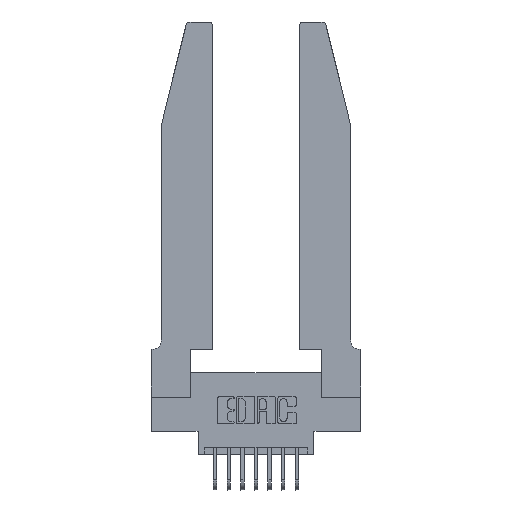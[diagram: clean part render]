
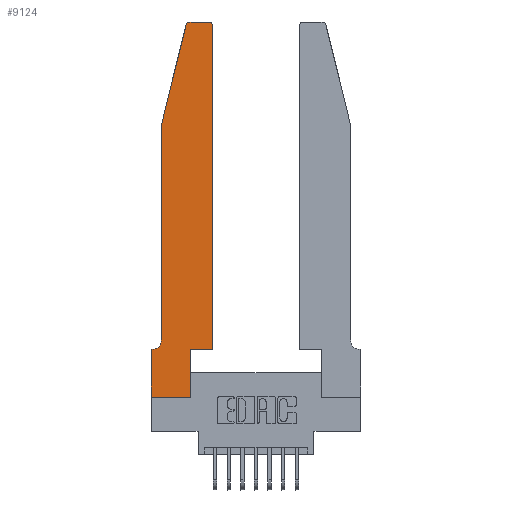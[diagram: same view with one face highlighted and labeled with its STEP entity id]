
A CAD part, top view. The second image highlights one B-rep face of the part: STEP entity #9124.
In plain terms, the highlighted planar face has unit normal (0, 0, 1).
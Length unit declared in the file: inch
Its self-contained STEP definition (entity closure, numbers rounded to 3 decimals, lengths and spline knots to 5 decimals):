
#321 = CARTESIAN_POINT ( 'NONE',  ( 0.0755, 2., 0.37 ) ) ;
#532 = DIRECTION ( 'NONE',  ( -0.239, -0.971, 0. ) ) ;
#691 = DIRECTION ( 'NONE',  ( 1., 0., 0. ) ) ;
#739 = FACE_OUTER_BOUND ( 'NONE', #866, .T. ) ;
#762 = ORIENTED_EDGE ( 'NONE', *, *, #8287, .T. ) ;
#866 = EDGE_LOOP ( 'NONE', ( #4754, #2908, #10912, #8141, #12727, #3979, #762, #2151, #1690, #1824, #6957, #2528 ) ) ;
#906 = EDGE_CURVE ( 'NONE', #6568, #2454, #1935, .T. ) ;
#1065 = AXIS2_PLACEMENT_3D ( 'NONE', #1657, #1554, #691 ) ;
#1554 = DIRECTION ( 'NONE',  ( 0., 0., 1. ) ) ;
#1657 = CARTESIAN_POINT ( 'NONE',  ( 0.284, 2.72, 0.37 ) ) ;
#1690 = ORIENTED_EDGE ( 'NONE', *, *, #4839, .T. ) ;
#1824 = ORIENTED_EDGE ( 'NONE', *, *, #3518, .T. ) ;
#1935 = LINE ( 'NONE', #15630, #15192 ) ;
#2151 = ORIENTED_EDGE ( 'NONE', *, *, #6370, .T. ) ;
#2232 = DIRECTION ( 'NONE',  ( 0., 0., -1. ) ) ;
#2344 = DIRECTION ( 'NONE',  ( 1., 0., 0. ) ) ;
#2454 = VERTEX_POINT ( 'NONE', #4902 ) ;
#2528 = ORIENTED_EDGE ( 'NONE', *, *, #13928, .T. ) ;
#2529 = EDGE_CURVE ( 'NONE', #5064, #13050, #14979, .T. ) ;
#2542 = AXIS2_PLACEMENT_3D ( 'NONE', #3660, #16476, #8797 ) ;
#2670 = LINE ( 'NONE', #3162, #9095 ) ;
#2908 = ORIENTED_EDGE ( 'NONE', *, *, #2529, .T. ) ;
#2967 = DIRECTION ( 'NONE',  ( 0., 0., 1. ) ) ;
#3162 = CARTESIAN_POINT ( 'NONE',  ( 0.0755, 2., 0.37 ) ) ;
#3518 = EDGE_CURVE ( 'NONE', #9784, #12158, #11514, .T. ) ;
#3660 = CARTESIAN_POINT ( 'NONE',  ( 0., 0.35, 0.37 ) ) ;
#3701 = LINE ( 'NONE', #15547, #13466 ) ;
#3979 = ORIENTED_EDGE ( 'NONE', *, *, #906, .T. ) ;
#3990 = DIRECTION ( 'NONE',  ( 1., 0., 0. ) ) ;
#4153 = LINE ( 'NONE', #8307, #13906 ) ;
#4227 = DIRECTION ( 'NONE',  ( 0., 1., 0. ) ) ;
#4754 = ORIENTED_EDGE ( 'NONE', *, *, #16108, .T. ) ;
#4839 = EDGE_CURVE ( 'NONE', #8522, #9784, #3701, .T. ) ;
#4902 = CARTESIAN_POINT ( 'NONE',  ( 0., 0.35, 0.37 ) ) ;
#5064 = VERTEX_POINT ( 'NONE', #5830 ) ;
#5167 = VECTOR ( 'NONE', #2344, 39.37008 ) ;
#5707 = VECTOR ( 'NONE', #6955, 39.37008 ) ;
#5830 = CARTESIAN_POINT ( 'NONE',  ( 0.284, 2.75, 0.37 ) ) ;
#5882 = LINE ( 'NONE', #12896, #12227 ) ;
#6125 = AXIS2_PLACEMENT_3D ( 'NONE', #9896, #2232, #11203 ) ;
#6370 = EDGE_CURVE ( 'NONE', #12316, #8522, #5882, .T. ) ;
#6496 = VERTEX_POINT ( 'NONE', #8105 ) ;
#6568 = VERTEX_POINT ( 'NONE', #15944 ) ;
#6630 = DIRECTION ( 'NONE',  ( 0., 1., 0. ) ) ;
#6821 = CARTESIAN_POINT ( 'NONE',  ( 0.4505, 0.35, 0.37 ) ) ;
#6955 = DIRECTION ( 'NONE',  ( 0., -1., 0. ) ) ;
#6957 = ORIENTED_EDGE ( 'NONE', *, *, #11340, .T. ) ;
#7007 = LINE ( 'NONE', #6821, #12957 ) ;
#7086 = CARTESIAN_POINT ( 'NONE',  ( 0.25487, 2.72718, 0.37 ) ) ;
#7095 = EDGE_CURVE ( 'NONE', #13050, #7576, #2670, .T. ) ;
#7122 = CARTESIAN_POINT ( 'NONE',  ( 0.0755, 0.42, 0.37 ) ) ;
#7249 = AXIS2_PLACEMENT_3D ( 'NONE', #10598, #2967, #11891 ) ;
#7576 = VERTEX_POINT ( 'NONE', #321 ) ;
#8105 = CARTESIAN_POINT ( 'NONE',  ( 0.4505, 2.72, 0.37 ) ) ;
#8141 = ORIENTED_EDGE ( 'NONE', *, *, #12514, .T. ) ;
#8287 = EDGE_CURVE ( 'NONE', #2454, #12316, #9082, .T. ) ;
#8307 = CARTESIAN_POINT ( 'NONE',  ( 0.0755, 2., 0.37 ) ) ;
#8459 = EDGE_CURVE ( 'NONE', #12044, #6568, #16489, .T. ) ;
#8522 = VERTEX_POINT ( 'NONE', #15077 ) ;
#8783 = DIRECTION ( 'NONE',  ( -1., 0., 0. ) ) ;
#8797 = DIRECTION ( 'NONE',  ( 1., 0., 0. ) ) ;
#8838 = DIRECTION ( 'NONE',  ( -1., 0., 0. ) ) ;
#9082 = LINE ( 'NONE', #15887, #5707 ) ;
#9095 = VECTOR ( 'NONE', #532, 39.37008 ) ;
#9124 = ADVANCED_FACE ( 'NONE', ( #739 ), #16419, .T. ) ;
#9158 = VECTOR ( 'NONE', #8783, 39.37008 ) ;
#9535 = VERTEX_POINT ( 'NONE', #13343 ) ;
#9577 = DIRECTION ( 'NONE',  ( 0., -1., 0. ) ) ;
#9784 = VERTEX_POINT ( 'NONE', #13885 ) ;
#9896 = CARTESIAN_POINT ( 'NONE',  ( 0.0055, 0.42, 0.37 ) ) ;
#10004 = CARTESIAN_POINT ( 'NONE',  ( 0.4505, 0.35, 0.37 ) ) ;
#10598 = CARTESIAN_POINT ( 'NONE',  ( 0.4205, 2.72, 0.37 ) ) ;
#10912 = ORIENTED_EDGE ( 'NONE', *, *, #7095, .T. ) ;
#11203 = DIRECTION ( 'NONE',  ( -1., 0., 0. ) ) ;
#11340 = EDGE_CURVE ( 'NONE', #12158, #6496, #7007, .T. ) ;
#11514 = LINE ( 'NONE', #10004, #5167 ) ;
#11891 = DIRECTION ( 'NONE',  ( 1., 0., 0. ) ) ;
#12044 = VERTEX_POINT ( 'NONE', #7122 ) ;
#12158 = VERTEX_POINT ( 'NONE', #13605 ) ;
#12178 = CIRCLE ( 'NONE', #7249, 0.03 ) ;
#12227 = VECTOR ( 'NONE', #3990, 39.37008 ) ;
#12316 = VERTEX_POINT ( 'NONE', #15248 ) ;
#12514 = EDGE_CURVE ( 'NONE', #7576, #12044, #4153, .T. ) ;
#12564 = CARTESIAN_POINT ( 'NONE',  ( 0.2605, 2.75, 0.37 ) ) ;
#12727 = ORIENTED_EDGE ( 'NONE', *, *, #8459, .T. ) ;
#12896 = CARTESIAN_POINT ( 'NONE',  ( 0., 0., 0.37 ) ) ;
#12957 = VECTOR ( 'NONE', #4227, 39.37008 ) ;
#13050 = VERTEX_POINT ( 'NONE', #7086 ) ;
#13343 = CARTESIAN_POINT ( 'NONE',  ( 0.4205, 2.75, 0.37 ) ) ;
#13466 = VECTOR ( 'NONE', #6630, 39.37008 ) ;
#13605 = CARTESIAN_POINT ( 'NONE',  ( 0.4505, 0.35, 0.37 ) ) ;
#13885 = CARTESIAN_POINT ( 'NONE',  ( 0.2865, 0.35, 0.37 ) ) ;
#13906 = VECTOR ( 'NONE', #9577, 39.37008 ) ;
#13928 = EDGE_CURVE ( 'NONE', #6496, #9535, #12178, .T. ) ;
#14979 = CIRCLE ( 'NONE', #1065, 0.03 ) ;
#15077 = CARTESIAN_POINT ( 'NONE',  ( 0.2865, 0., 0.37 ) ) ;
#15192 = VECTOR ( 'NONE', #8838, 39.37008 ) ;
#15248 = CARTESIAN_POINT ( 'NONE',  ( 0., 0., 0.37 ) ) ;
#15547 = CARTESIAN_POINT ( 'NONE',  ( 0.2865, 0.35, 0.37 ) ) ;
#15630 = CARTESIAN_POINT ( 'NONE',  ( 0.0755, 0.35, 0.37 ) ) ;
#15887 = CARTESIAN_POINT ( 'NONE',  ( 0., 0., 0.37 ) ) ;
#15944 = CARTESIAN_POINT ( 'NONE',  ( 0.0055, 0.35, 0.37 ) ) ;
#16108 = EDGE_CURVE ( 'NONE', #9535, #5064, #16371, .T. ) ;
#16371 = LINE ( 'NONE', #12564, #9158 ) ;
#16419 = PLANE ( 'NONE',  #2542 ) ;
#16476 = DIRECTION ( 'NONE',  ( 0., 0., 1. ) ) ;
#16489 = CIRCLE ( 'NONE', #6125, 0.07 ) ;
